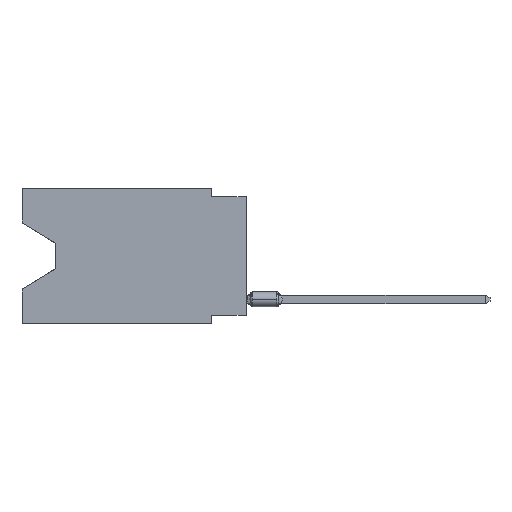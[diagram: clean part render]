
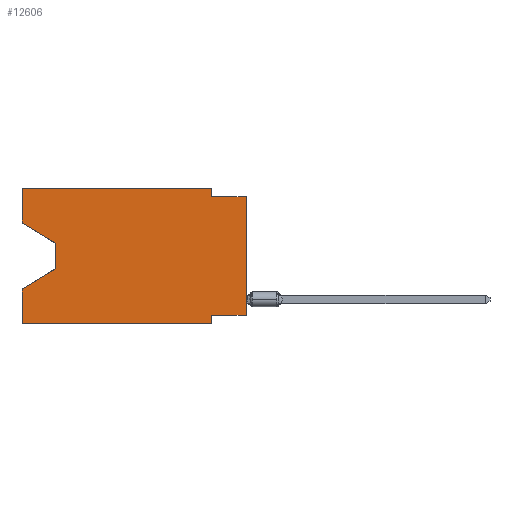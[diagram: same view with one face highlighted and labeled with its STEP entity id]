
A CAD part, left-side view. The second image highlights one B-rep face of the part: STEP entity #12606.
In plain terms, the highlighted planar face has unit normal (-1, 0, 0).
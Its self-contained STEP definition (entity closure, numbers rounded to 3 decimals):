
#126 = DIRECTION ( 'NONE',  ( 0., 0., -1. ) ) ;
#155 = CARTESIAN_POINT ( 'NONE',  ( 0., 13.97, -4.013 ) ) ;
#227 = PLANE ( 'NONE',  #3773 ) ;
#276 = VECTOR ( 'NONE', #13092, 1000. ) ;
#555 = LINE ( 'NONE', #3517, #8522 ) ;
#827 = CARTESIAN_POINT ( 'NONE',  ( 0., 2.54, -0.635 ) ) ;
#1280 = ORIENTED_EDGE ( 'NONE', *, *, #16442, .T. ) ;
#1291 = DIRECTION ( 'NONE',  ( 0., -1., 0. ) ) ;
#1301 = CARTESIAN_POINT ( 'NONE',  ( 0., 0., -0.635 ) ) ;
#1539 = ORIENTED_EDGE ( 'NONE', *, *, #10487, .F. ) ;
#1557 = VERTEX_POINT ( 'NONE', #15009 ) ;
#1572 = ORIENTED_EDGE ( 'NONE', *, *, #3699, .F. ) ;
#1652 = ORIENTED_EDGE ( 'NONE', *, *, #12825, .F. ) ;
#1861 = CARTESIAN_POINT ( 'NONE',  ( 0., 16.383, 0. ) ) ;
#1927 = CARTESIAN_POINT ( 'NONE',  ( 0., 2.54, -9.906 ) ) ;
#2572 = LINE ( 'NONE', #14974, #3772 ) ;
#2684 = CARTESIAN_POINT ( 'NONE',  ( 0., 16.383, -9.906 ) ) ;
#2833 = EDGE_CURVE ( 'NONE', #1557, #16951, #9724, .T. ) ;
#2835 = VECTOR ( 'NONE', #8729, 1000. ) ;
#2932 = CARTESIAN_POINT ( 'NONE',  ( 0., 2.54, 0. ) ) ;
#3042 = VECTOR ( 'NONE', #16313, 1000. ) ;
#3375 = LINE ( 'NONE', #9223, #3042 ) ;
#3517 = CARTESIAN_POINT ( 'NONE',  ( 0., 0., -9.271 ) ) ;
#3582 = EDGE_CURVE ( 'NONE', #8052, #13952, #17452, .T. ) ;
#3648 = LINE ( 'NONE', #9317, #8525 ) ;
#3662 = CARTESIAN_POINT ( 'NONE',  ( 0., 0., -9.271 ) ) ;
#3699 = EDGE_CURVE ( 'NONE', #6912, #8052, #11064, .T. ) ;
#3710 = VECTOR ( 'NONE', #7078, 1000. ) ;
#3772 = VECTOR ( 'NONE', #7971, 1000. ) ;
#3773 = AXIS2_PLACEMENT_3D ( 'NONE', #4396, #10044, #126 ) ;
#4151 = ORIENTED_EDGE ( 'NONE', *, *, #5222, .F. ) ;
#4157 = VERTEX_POINT ( 'NONE', #1301 ) ;
#4396 = CARTESIAN_POINT ( 'NONE',  ( 0., 16.383, 0. ) ) ;
#4451 = CARTESIAN_POINT ( 'NONE',  ( 0., 16.383, -2.546 ) ) ;
#4599 = VECTOR ( 'NONE', #8291, 1000. ) ;
#4700 = LINE ( 'NONE', #8879, #9895 ) ;
#5002 = ORIENTED_EDGE ( 'NONE', *, *, #2833, .T. ) ;
#5222 = EDGE_CURVE ( 'NONE', #14342, #4157, #3375, .T. ) ;
#5438 = LINE ( 'NONE', #2932, #6114 ) ;
#5791 = ORIENTED_EDGE ( 'NONE', *, *, #9573, .T. ) ;
#5959 = CARTESIAN_POINT ( 'NONE',  ( 0., 13.97, -4.013 ) ) ;
#6114 = VECTOR ( 'NONE', #11098, 1000. ) ;
#6655 = DIRECTION ( 'NONE',  ( 0., 1., 0. ) ) ;
#6912 = VERTEX_POINT ( 'NONE', #4451 ) ;
#6942 = VECTOR ( 'NONE', #1291, 1000. ) ;
#7003 = ORIENTED_EDGE ( 'NONE', *, *, #14458, .T. ) ;
#7058 = EDGE_CURVE ( 'NONE', #1557, #17743, #17408, .T. ) ;
#7078 = DIRECTION ( 'NONE',  ( 0., 0., -1. ) ) ;
#7459 = CARTESIAN_POINT ( 'NONE',  ( 0., 0., 0. ) ) ;
#7971 = DIRECTION ( 'NONE',  ( 0., 0.855, -0.519 ) ) ;
#8052 = VERTEX_POINT ( 'NONE', #16287 ) ;
#8281 = CARTESIAN_POINT ( 'NONE',  ( 0., 2.54, -9.271 ) ) ;
#8291 = DIRECTION ( 'NONE',  ( 0., 0., 1. ) ) ;
#8476 = LINE ( 'NONE', #5959, #3710 ) ;
#8522 = VECTOR ( 'NONE', #6655, 1000. ) ;
#8525 = VECTOR ( 'NONE', #10614, 1000. ) ;
#8729 = DIRECTION ( 'NONE',  ( 0., 0., 1. ) ) ;
#8879 = CARTESIAN_POINT ( 'NONE',  ( 0., 16.383, -2.546 ) ) ;
#8898 = VERTEX_POINT ( 'NONE', #16029 ) ;
#9223 = CARTESIAN_POINT ( 'NONE',  ( 0., 0., -0.635 ) ) ;
#9317 = CARTESIAN_POINT ( 'NONE',  ( 0., 2.54, -9.906 ) ) ;
#9573 = EDGE_CURVE ( 'NONE', #6912, #18005, #4700, .T. ) ;
#9655 = VERTEX_POINT ( 'NONE', #3662 ) ;
#9724 = LINE ( 'NONE', #2684, #6942 ) ;
#9829 = CARTESIAN_POINT ( 'NONE',  ( 0., 16.383, -7.36 ) ) ;
#9895 = VECTOR ( 'NONE', #14495, 1000. ) ;
#10038 = EDGE_CURVE ( 'NONE', #18005, #8898, #8476, .T. ) ;
#10044 = DIRECTION ( 'NONE',  ( 1., 0., 0. ) ) ;
#10487 = EDGE_CURVE ( 'NONE', #9655, #12883, #555, .T. ) ;
#10614 = DIRECTION ( 'NONE',  ( 0., 0., -1. ) ) ;
#10626 = DIRECTION ( 'NONE',  ( 0., -1., 0. ) ) ;
#11064 = LINE ( 'NONE', #15128, #4599 ) ;
#11098 = DIRECTION ( 'NONE',  ( 0., 0., -1. ) ) ;
#11440 = FACE_OUTER_BOUND ( 'NONE', #12147, .T. ) ;
#12016 = VECTOR ( 'NONE', #10626, 1000. ) ;
#12108 = CARTESIAN_POINT ( 'NONE',  ( 0., 16.383, 0. ) ) ;
#12143 = EDGE_CURVE ( 'NONE', #13952, #14342, #5438, .T. ) ;
#12147 = EDGE_LOOP ( 'NONE', ( #5791, #14976, #7003, #15730, #5002, #1652, #1539, #1280, #4151, #12761, #18258, #1572 ) ) ;
#12606 = ADVANCED_FACE ( 'NONE', ( #11440 ), #227, .F. ) ;
#12761 = ORIENTED_EDGE ( 'NONE', *, *, #12143, .F. ) ;
#12825 = EDGE_CURVE ( 'NONE', #12883, #16951, #3648, .T. ) ;
#12883 = VERTEX_POINT ( 'NONE', #8281 ) ;
#13092 = DIRECTION ( 'NONE',  ( 0., 0., 1. ) ) ;
#13952 = VERTEX_POINT ( 'NONE', #14467 ) ;
#14342 = VERTEX_POINT ( 'NONE', #827 ) ;
#14458 = EDGE_CURVE ( 'NONE', #8898, #17743, #2572, .T. ) ;
#14467 = CARTESIAN_POINT ( 'NONE',  ( 0., 2.54, 0. ) ) ;
#14495 = DIRECTION ( 'NONE',  ( 0., -0.855, -0.519 ) ) ;
#14974 = CARTESIAN_POINT ( 'NONE',  ( 0., 13.97, -5.893 ) ) ;
#14976 = ORIENTED_EDGE ( 'NONE', *, *, #10038, .T. ) ;
#15009 = CARTESIAN_POINT ( 'NONE',  ( 0., 16.383, -9.906 ) ) ;
#15128 = CARTESIAN_POINT ( 'NONE',  ( 0., 16.383, 0. ) ) ;
#15730 = ORIENTED_EDGE ( 'NONE', *, *, #7058, .F. ) ;
#16029 = CARTESIAN_POINT ( 'NONE',  ( 0., 13.97, -5.893 ) ) ;
#16287 = CARTESIAN_POINT ( 'NONE',  ( 0., 16.383, 0. ) ) ;
#16313 = DIRECTION ( 'NONE',  ( 0., -1., 0. ) ) ;
#16442 = EDGE_CURVE ( 'NONE', #9655, #4157, #17521, .T. ) ;
#16951 = VERTEX_POINT ( 'NONE', #1927 ) ;
#17408 = LINE ( 'NONE', #1861, #2835 ) ;
#17452 = LINE ( 'NONE', #12108, #12016 ) ;
#17521 = LINE ( 'NONE', #7459, #276 ) ;
#17743 = VERTEX_POINT ( 'NONE', #9829 ) ;
#18005 = VERTEX_POINT ( 'NONE', #155 ) ;
#18258 = ORIENTED_EDGE ( 'NONE', *, *, #3582, .F. ) ;
